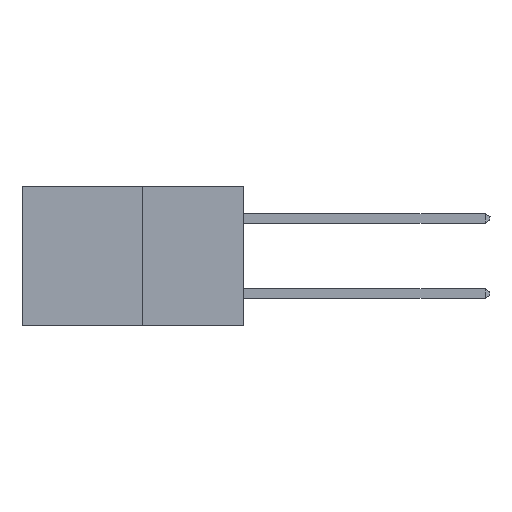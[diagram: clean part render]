
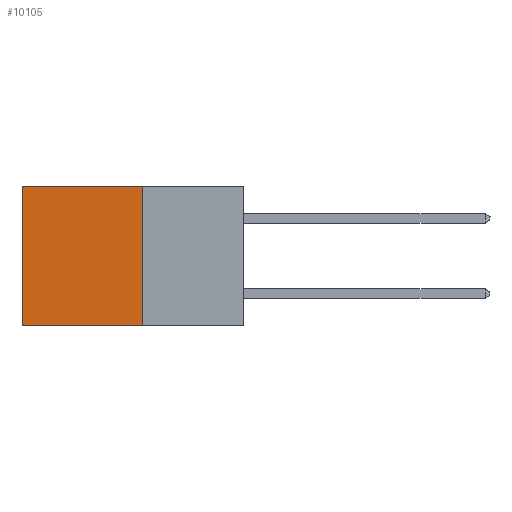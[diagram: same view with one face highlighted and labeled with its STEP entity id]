
A CAD part, left-side view. The second image highlights one B-rep face of the part: STEP entity #10105.
In plain terms, the highlighted planar face has unit normal (-1, 0, 0).
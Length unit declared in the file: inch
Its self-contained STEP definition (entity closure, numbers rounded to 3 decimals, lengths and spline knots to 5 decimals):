
#173 = EDGE_CURVE ( 'NONE', #5194, #385, #3568, .T. ) ;
#385 = VERTEX_POINT ( 'NONE', #1594 ) ;
#401 = LINE ( 'NONE', #8037, #2340 ) ;
#788 = CARTESIAN_POINT ( 'NONE',  ( 0.277, 0.27, -0.37 ) ) ;
#1028 = ORIENTED_EDGE ( 'NONE', *, *, #8794, .T. ) ;
#1131 = DIRECTION ( 'NONE',  ( 0., 1., 0. ) ) ;
#1366 = VECTOR ( 'NONE', #1131, 39.37008 ) ;
#1594 = CARTESIAN_POINT ( 'NONE',  ( 0.277, 0.27, -0.37 ) ) ;
#1683 = DIRECTION ( 'NONE',  ( 0., 1., 0. ) ) ;
#1725 = DIRECTION ( 'NONE',  ( 1., 0., 0. ) ) ;
#1906 = EDGE_CURVE ( 'NONE', #385, #2524, #8444, .T. ) ;
#1956 = EDGE_LOOP ( 'NONE', ( #10412, #3944, #10762, #1028 ) ) ;
#2340 = VECTOR ( 'NONE', #7098, 39.37008 ) ;
#2524 = VERTEX_POINT ( 'NONE', #9684 ) ;
#2570 = CARTESIAN_POINT ( 'NONE',  ( 0.277, 0.27, -0.37 ) ) ;
#2866 = VERTEX_POINT ( 'NONE', #6316 ) ;
#3568 = LINE ( 'NONE', #11726, #10421 ) ;
#3654 = FACE_OUTER_BOUND ( 'NONE', #1956, .T. ) ;
#3944 = ORIENTED_EDGE ( 'NONE', *, *, #1906, .F. ) ;
#5063 = VECTOR ( 'NONE', #1683, 39.37008 ) ;
#5194 = VERTEX_POINT ( 'NONE', #6226 ) ;
#6226 = CARTESIAN_POINT ( 'NONE',  ( 0.277, 0.27, 0. ) ) ;
#6316 = CARTESIAN_POINT ( 'NONE',  ( 0.277, 0.59, 0. ) ) ;
#6525 = PLANE ( 'NONE',  #9563 ) ;
#6795 = DIRECTION ( 'NONE',  ( 0., 0., -1. ) ) ;
#6898 = CARTESIAN_POINT ( 'NONE',  ( 0.277, 0.27, 0. ) ) ;
#7061 = EDGE_CURVE ( 'NONE', #2866, #2524, #401, .T. ) ;
#7098 = DIRECTION ( 'NONE',  ( 0., 0., -1. ) ) ;
#8037 = CARTESIAN_POINT ( 'NONE',  ( 0.277, 0.59, -0.37 ) ) ;
#8434 = DIRECTION ( 'NONE',  ( 0., 0., -1. ) ) ;
#8444 = LINE ( 'NONE', #2570, #5063 ) ;
#8794 = EDGE_CURVE ( 'NONE', #5194, #2866, #8996, .T. ) ;
#8996 = LINE ( 'NONE', #6898, #1366 ) ;
#9563 = AXIS2_PLACEMENT_3D ( 'NONE', #788, #1725, #8434 ) ;
#9684 = CARTESIAN_POINT ( 'NONE',  ( 0.277, 0.59, -0.37 ) ) ;
#10105 = ADVANCED_FACE ( 'NONE', ( #3654 ), #6525, .F. ) ;
#10412 = ORIENTED_EDGE ( 'NONE', *, *, #7061, .T. ) ;
#10421 = VECTOR ( 'NONE', #6795, 39.37008 ) ;
#10762 = ORIENTED_EDGE ( 'NONE', *, *, #173, .F. ) ;
#11726 = CARTESIAN_POINT ( 'NONE',  ( 0.277, 0.27, -0.37 ) ) ;
